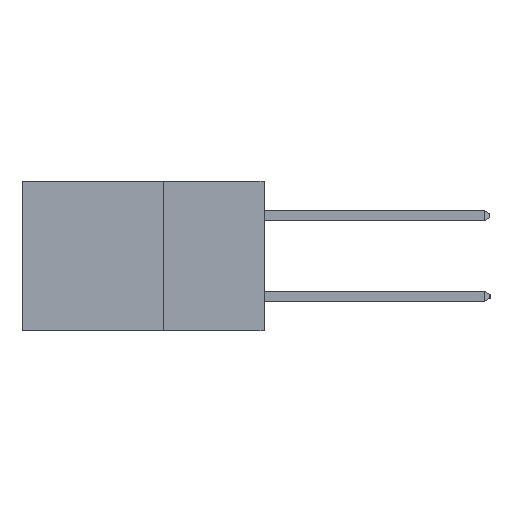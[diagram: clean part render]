
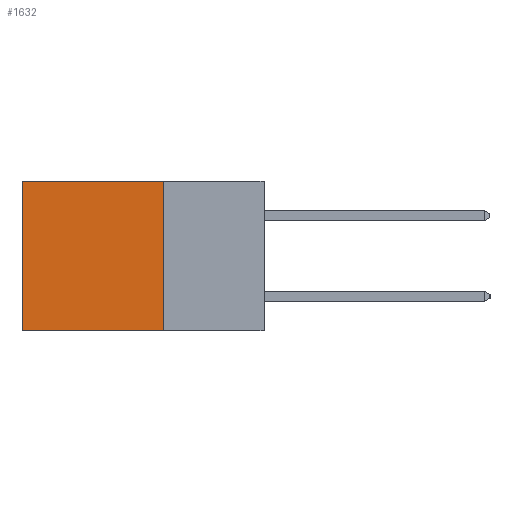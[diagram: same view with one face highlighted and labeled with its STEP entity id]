
A CAD part, left-side view. The second image highlights one B-rep face of the part: STEP entity #1632.
In plain terms, the highlighted planar face has unit normal (-1, 0, 0).
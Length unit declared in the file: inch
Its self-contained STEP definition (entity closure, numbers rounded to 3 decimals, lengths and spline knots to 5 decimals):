
#756 = VECTOR ( 'NONE', #10333, 39.37008 ) ;
#1032 = EDGE_CURVE ( 'NONE', #6444, #8118, #2843, .T. ) ;
#1151 = CARTESIAN_POINT ( 'NONE',  ( 0.2615, 0.25, -0.37 ) ) ;
#1481 = AXIS2_PLACEMENT_3D ( 'NONE', #9433, #9115, #9402 ) ;
#1566 = VECTOR ( 'NONE', #3118, 39.37008 ) ;
#1632 = ADVANCED_FACE ( 'NONE', ( #5717 ), #9192, .F. ) ;
#1830 = LINE ( 'NONE', #8111, #1566 ) ;
#2843 = LINE ( 'NONE', #3026, #4796 ) ;
#2915 = CARTESIAN_POINT ( 'NONE',  ( 0.2615, 0.25, 0. ) ) ;
#3018 = ORIENTED_EDGE ( 'NONE', *, *, #3315, .T. ) ;
#3026 = CARTESIAN_POINT ( 'NONE',  ( 0.2615, 0.25, -0.37 ) ) ;
#3053 = LINE ( 'NONE', #2915, #756 ) ;
#3118 = DIRECTION ( 'NONE',  ( 0., 0., -1. ) ) ;
#3143 = EDGE_CURVE ( 'NONE', #9313, #6444, #7635, .T. ) ;
#3315 = EDGE_CURVE ( 'NONE', #5145, #8118, #1830, .T. ) ;
#3468 = VECTOR ( 'NONE', #7899, 39.37008 ) ;
#3833 = EDGE_CURVE ( 'NONE', #9313, #5145, #3053, .T. ) ;
#4017 = ORIENTED_EDGE ( 'NONE', *, *, #1032, .F. ) ;
#4276 = CARTESIAN_POINT ( 'NONE',  ( 0.2615, 0.25, -0.37 ) ) ;
#4796 = VECTOR ( 'NONE', #6728, 39.37008 ) ;
#5145 = VERTEX_POINT ( 'NONE', #9640 ) ;
#5573 = EDGE_LOOP ( 'NONE', ( #3018, #4017, #7384, #7615 ) ) ;
#5717 = FACE_OUTER_BOUND ( 'NONE', #5573, .T. ) ;
#6444 = VERTEX_POINT ( 'NONE', #4276 ) ;
#6728 = DIRECTION ( 'NONE',  ( 0., 1., 0. ) ) ;
#7384 = ORIENTED_EDGE ( 'NONE', *, *, #3143, .F. ) ;
#7615 = ORIENTED_EDGE ( 'NONE', *, *, #3833, .T. ) ;
#7635 = LINE ( 'NONE', #1151, #3468 ) ;
#7899 = DIRECTION ( 'NONE',  ( 0., 0., -1. ) ) ;
#8111 = CARTESIAN_POINT ( 'NONE',  ( 0.2615, 0.6, -0.37 ) ) ;
#8118 = VERTEX_POINT ( 'NONE', #10464 ) ;
#9115 = DIRECTION ( 'NONE',  ( 1., 0., 0. ) ) ;
#9192 = PLANE ( 'NONE',  #1481 ) ;
#9313 = VERTEX_POINT ( 'NONE', #10101 ) ;
#9402 = DIRECTION ( 'NONE',  ( 0., 0., -1. ) ) ;
#9433 = CARTESIAN_POINT ( 'NONE',  ( 0.2615, 0.25, -0.37 ) ) ;
#9640 = CARTESIAN_POINT ( 'NONE',  ( 0.2615, 0.6, 0. ) ) ;
#10101 = CARTESIAN_POINT ( 'NONE',  ( 0.2615, 0.25, 0. ) ) ;
#10333 = DIRECTION ( 'NONE',  ( 0., 1., 0. ) ) ;
#10464 = CARTESIAN_POINT ( 'NONE',  ( 0.2615, 0.6, -0.37 ) ) ;
